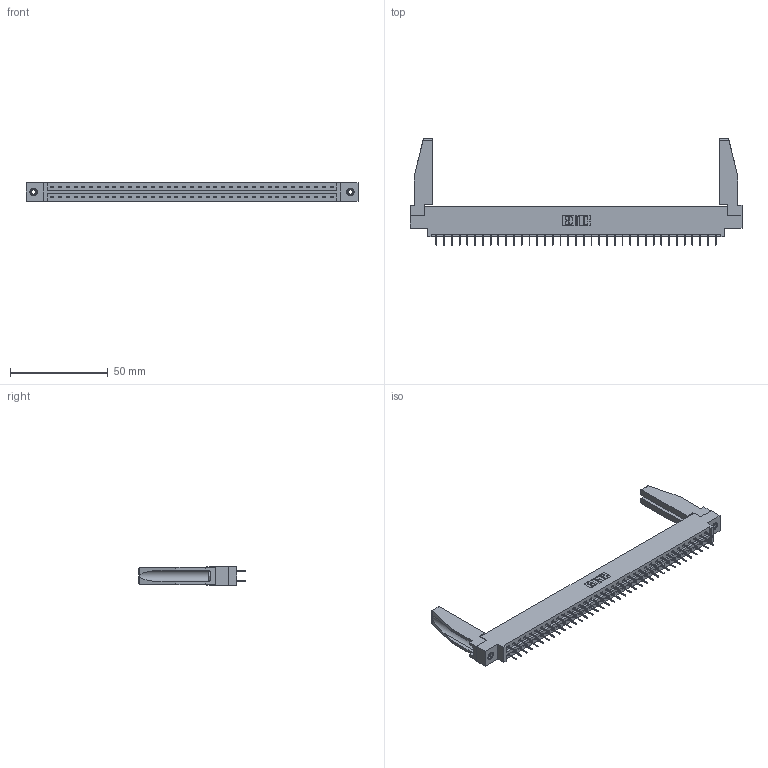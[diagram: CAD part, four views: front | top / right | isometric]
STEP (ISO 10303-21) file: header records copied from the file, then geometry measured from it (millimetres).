
FILE_DESCRIPTION (( 'STEP AP203' ), '1' );
FILE_NAME ('337-074-524-878.STEP', '2019-10-15T12:25:55', ( '' ), ( '' ), 'SwSTEP 2.0', 'SolidWorks 2016', '' );
FILE_SCHEMA (( 'CONFIG_CONTROL_DESIGN' ));
Length unit declared in the file: inch
Products named in the file (5): 337-074-524-878; 337 Part_0.170 Offset - 0.156 Dia-TI; 345-292-001_345-293-124; 345-250-001_345-250-001-102; 307-220-078
Assembly tree (79 placements, depth 2):
  337-074-524-878
    337 Part_0.170 Offset - 0.156 Dia-TI
    345-292-001_345-293-124  x74
    345-250-001_345-250-001-102  x2
    307-220-078  x2
Bounding box: 169.62 x 54.49 x 9.4 mm (x, y, z)
Volume: 21573.3 mm3; surface area: 23417.1 mm2
Topology: 79 solids, 79 shells, 4540 faces, 12863 edges, 8270 vertices
Faces by surface type: plane 3414, cylinder 1110, cone 12, torus 4
Entity records: 31980 total; most frequent: CARTESIAN_POINT 5392, ORIENTED_EDGE 5284, DIRECTION 4602, EDGE_CURVE 2642, VECTOR 2480, LINE 2480, VERTEX_POINT 1752, AXIS2_PLACEMENT_3D 1061
